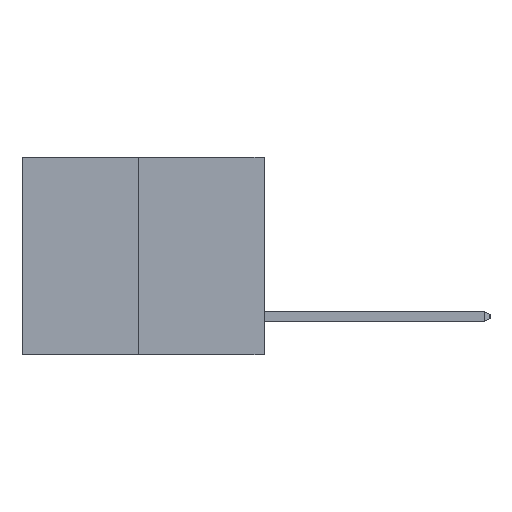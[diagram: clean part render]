
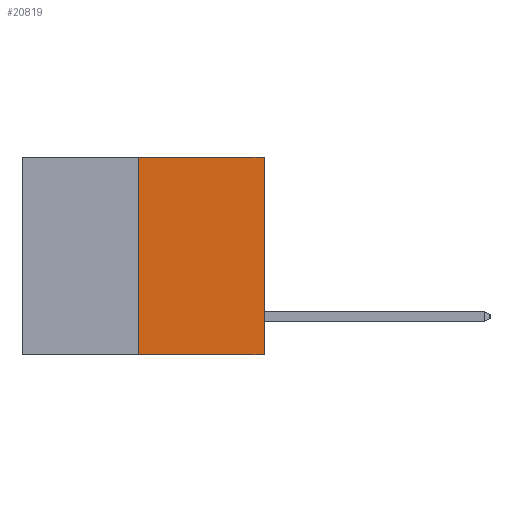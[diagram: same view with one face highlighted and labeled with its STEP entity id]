
A CAD part, left-side view. The second image highlights one B-rep face of the part: STEP entity #20819.
In plain terms, the highlighted planar face has unit normal (-1, 0, 0).
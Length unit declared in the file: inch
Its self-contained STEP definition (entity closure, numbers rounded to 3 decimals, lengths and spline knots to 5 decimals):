
#3877 = DIRECTION ( 'NONE',  ( 0., 0., -1. ) ) ;
#4012 = ORIENTED_EDGE ( 'NONE', *, *, #5450, .F. ) ;
#4102 = LINE ( 'NONE', #9028, #11133 ) ;
#4192 = DIRECTION ( 'NONE',  ( 0., 0., 1. ) ) ;
#4230 = CARTESIAN_POINT ( 'NONE',  ( 0., 0.312, -0.49 ) ) ;
#5450 = EDGE_CURVE ( 'NONE', #16778, #18722, #8115, .T. ) ;
#5738 = DIRECTION ( 'NONE',  ( 0., -1., 0. ) ) ;
#6077 = VERTEX_POINT ( 'NONE', #20160 ) ;
#7853 = VECTOR ( 'NONE', #5738, 39.37008 ) ;
#7920 = CARTESIAN_POINT ( 'NONE',  ( 0., 0., -0.49 ) ) ;
#8115 = LINE ( 'NONE', #25498, #12504 ) ;
#8662 = ORIENTED_EDGE ( 'NONE', *, *, #22663, .T. ) ;
#9028 = CARTESIAN_POINT ( 'NONE',  ( 0., 0., 0. ) ) ;
#11133 = VECTOR ( 'NONE', #4192, 39.37008 ) ;
#11583 = DIRECTION ( 'NONE',  ( 0., 0., 1. ) ) ;
#12504 = VECTOR ( 'NONE', #11583, 39.37008 ) ;
#12607 = ORIENTED_EDGE ( 'NONE', *, *, #17659, .T. ) ;
#12793 = CARTESIAN_POINT ( 'NONE',  ( 0., 0.312, 0. ) ) ;
#13389 = VERTEX_POINT ( 'NONE', #7920 ) ;
#13472 = DIRECTION ( 'NONE',  ( 1., 0., 0. ) ) ;
#13711 = CARTESIAN_POINT ( 'NONE',  ( 0., 0.6, -0.49 ) ) ;
#14737 = ORIENTED_EDGE ( 'NONE', *, *, #27088, .F. ) ;
#15645 = CARTESIAN_POINT ( 'NONE',  ( 0., 0.6, 0. ) ) ;
#16133 = AXIS2_PLACEMENT_3D ( 'NONE', #15645, #13472, #3877 ) ;
#16288 = DIRECTION ( 'NONE',  ( 0., -1., 0. ) ) ;
#16778 = VERTEX_POINT ( 'NONE', #4230 ) ;
#17546 = CARTESIAN_POINT ( 'NONE',  ( 0., 0.6, 0. ) ) ;
#17659 = EDGE_CURVE ( 'NONE', #16778, #13389, #22343, .T. ) ;
#18722 = VERTEX_POINT ( 'NONE', #12793 ) ;
#19946 = FACE_OUTER_BOUND ( 'NONE', #30622, .T. ) ;
#20160 = CARTESIAN_POINT ( 'NONE',  ( 0., 0., 0. ) ) ;
#20819 = ADVANCED_FACE ( 'NONE', ( #19946 ), #25122, .F. ) ;
#21197 = VECTOR ( 'NONE', #16288, 39.37008 ) ;
#22343 = LINE ( 'NONE', #13711, #21197 ) ;
#22663 = EDGE_CURVE ( 'NONE', #13389, #6077, #4102, .T. ) ;
#25122 = PLANE ( 'NONE',  #16133 ) ;
#25498 = CARTESIAN_POINT ( 'NONE',  ( 0., 0.312, -0.49 ) ) ;
#26389 = LINE ( 'NONE', #17546, #7853 ) ;
#27088 = EDGE_CURVE ( 'NONE', #18722, #6077, #26389, .T. ) ;
#30622 = EDGE_LOOP ( 'NONE', ( #4012, #12607, #8662, #14737 ) ) ;
